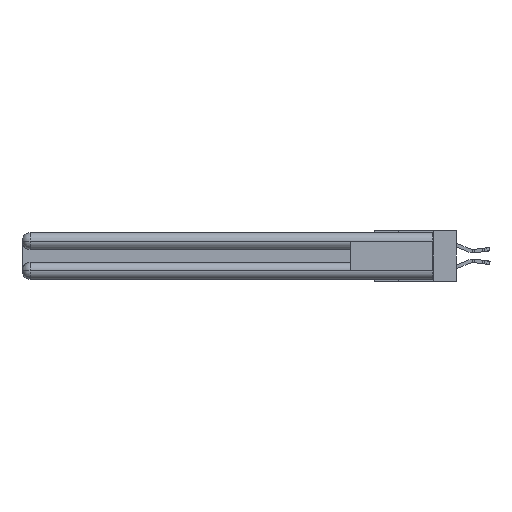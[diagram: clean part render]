
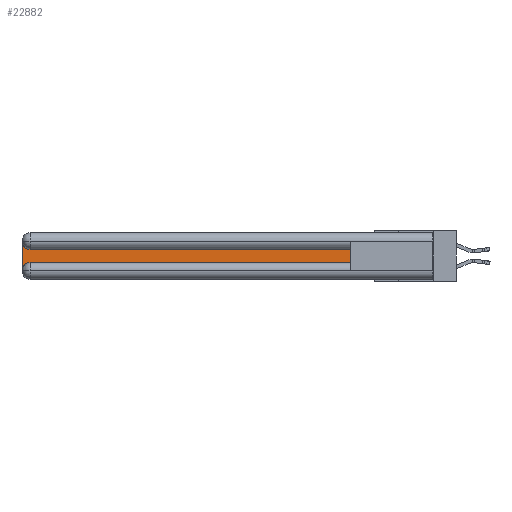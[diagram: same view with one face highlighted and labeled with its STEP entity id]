
A CAD part, left-side view. The second image highlights one B-rep face of the part: STEP entity #22882.
In plain terms, the highlighted planar face has unit normal (-1, 0, 0).
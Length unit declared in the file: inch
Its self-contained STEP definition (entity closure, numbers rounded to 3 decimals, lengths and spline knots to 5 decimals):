
#1535 = EDGE_CURVE ( 'NONE', #14354, #19433, #33026, .T. ) ;
#1790 = DIRECTION ( 'NONE',  ( 0., 0., -1. ) ) ;
#3953 = CARTESIAN_POINT ( 'NONE',  ( 0.075, 0.6, -0.2175 ) ) ;
#4607 = PLANE ( 'NONE',  #10097 ) ;
#4681 = CARTESIAN_POINT ( 'NONE',  ( 0.075, 3., -0.2775 ) ) ;
#4771 = ORIENTED_EDGE ( 'NONE', *, *, #23513, .T. ) ;
#5624 = EDGE_CURVE ( 'NONE', #26130, #15799, #15054, .T. ) ;
#5793 = CARTESIAN_POINT ( 'NONE',  ( 0.075, 3., -0.2175 ) ) ;
#6012 = CARTESIAN_POINT ( 'NONE',  ( 0.075, 2.94, -0.1225 ) ) ;
#7010 = ORIENTED_EDGE ( 'NONE', *, *, #27846, .T. ) ;
#7017 = ORIENTED_EDGE ( 'NONE', *, *, #33720, .T. ) ;
#7089 = EDGE_LOOP ( 'NONE', ( #18222, #9932, #7010, #32915, #7017, #4771 ) ) ;
#9932 = ORIENTED_EDGE ( 'NONE', *, *, #1535, .T. ) ;
#10097 = AXIS2_PLACEMENT_3D ( 'NONE', #17580, #15124, #1790 ) ;
#10135 = FACE_OUTER_BOUND ( 'NONE', #7089, .T. ) ;
#13434 = DIRECTION ( 'NONE',  ( 0., 0., 1. ) ) ;
#13603 = DIRECTION ( 'NONE',  ( 1., 0., 0. ) ) ;
#14354 = VERTEX_POINT ( 'NONE', #6012 ) ;
#15054 = CIRCLE ( 'NONE', #31531, 0.06 ) ;
#15124 = DIRECTION ( 'NONE',  ( 1., 0., 0. ) ) ;
#15157 = LINE ( 'NONE', #31678, #21201 ) ;
#15670 = CARTESIAN_POINT ( 'NONE',  ( 0.075, 0.6, -0.1225 ) ) ;
#15799 = VERTEX_POINT ( 'NONE', #23561 ) ;
#15833 = CARTESIAN_POINT ( 'NONE',  ( 0.075, 3., -0.0625 ) ) ;
#17580 = CARTESIAN_POINT ( 'NONE',  ( 0.075, 3., -0.1225 ) ) ;
#17692 = VECTOR ( 'NONE', #29535, 39.37008 ) ;
#18222 = ORIENTED_EDGE ( 'NONE', *, *, #21505, .T. ) ;
#19433 = VERTEX_POINT ( 'NONE', #15833 ) ;
#20802 = DIRECTION ( 'NONE',  ( 0., 0., -1. ) ) ;
#20901 = VERTEX_POINT ( 'NONE', #15670 ) ;
#21021 = DIRECTION ( 'NONE',  ( 1., 0., 0. ) ) ;
#21118 = CARTESIAN_POINT ( 'NONE',  ( 0.075, 2.94, -0.0625 ) ) ;
#21201 = VECTOR ( 'NONE', #13434, 39.37008 ) ;
#21505 = EDGE_CURVE ( 'NONE', #20901, #14354, #27733, .T. ) ;
#21825 = DIRECTION ( 'NONE',  ( 0., -1., 0. ) ) ;
#22430 = CARTESIAN_POINT ( 'NONE',  ( 0.075, 0.6, -0.1225 ) ) ;
#22816 = VERTEX_POINT ( 'NONE', #25239 ) ;
#22882 = ADVANCED_FACE ( 'NONE', ( #10135 ), #4607, .F. ) ;
#23513 = EDGE_CURVE ( 'NONE', #22816, #20901, #15157, .T. ) ;
#23561 = CARTESIAN_POINT ( 'NONE',  ( 0.075, 2.94, -0.2175 ) ) ;
#23618 = VECTOR ( 'NONE', #21825, 39.37008 ) ;
#25239 = CARTESIAN_POINT ( 'NONE',  ( 0.075, 0.6, -0.2175 ) ) ;
#26130 = VERTEX_POINT ( 'NONE', #4681 ) ;
#27733 = LINE ( 'NONE', #22430, #28932 ) ;
#27846 = EDGE_CURVE ( 'NONE', #19433, #26130, #31584, .T. ) ;
#28932 = VECTOR ( 'NONE', #30095, 39.37008 ) ;
#29535 = DIRECTION ( 'NONE',  ( 0., 0., -1. ) ) ;
#29575 = CARTESIAN_POINT ( 'NONE',  ( 0.075, 2.94, -0.2775 ) ) ;
#30095 = DIRECTION ( 'NONE',  ( 0., 1., 0. ) ) ;
#30618 = LINE ( 'NONE', #3953, #23618 ) ;
#31250 = AXIS2_PLACEMENT_3D ( 'NONE', #21118, #21021, #20802 ) ;
#31531 = AXIS2_PLACEMENT_3D ( 'NONE', #29575, #13603, #32083 ) ;
#31584 = LINE ( 'NONE', #5793, #17692 ) ;
#31678 = CARTESIAN_POINT ( 'NONE',  ( 0.075, 0.6, -0.2175 ) ) ;
#32083 = DIRECTION ( 'NONE',  ( 0., 0., -1. ) ) ;
#32915 = ORIENTED_EDGE ( 'NONE', *, *, #5624, .T. ) ;
#33026 = CIRCLE ( 'NONE', #31250, 0.06 ) ;
#33720 = EDGE_CURVE ( 'NONE', #15799, #22816, #30618, .T. ) ;
